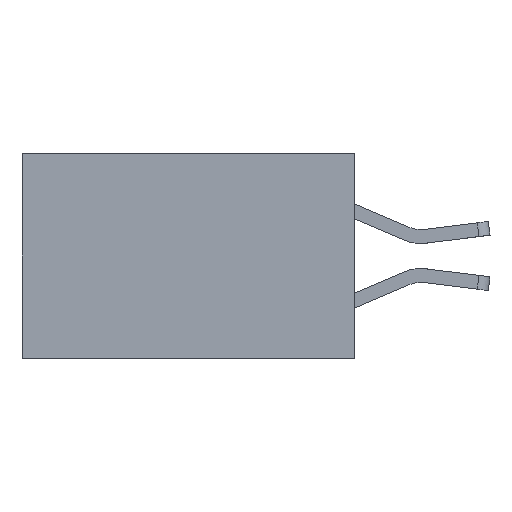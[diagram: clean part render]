
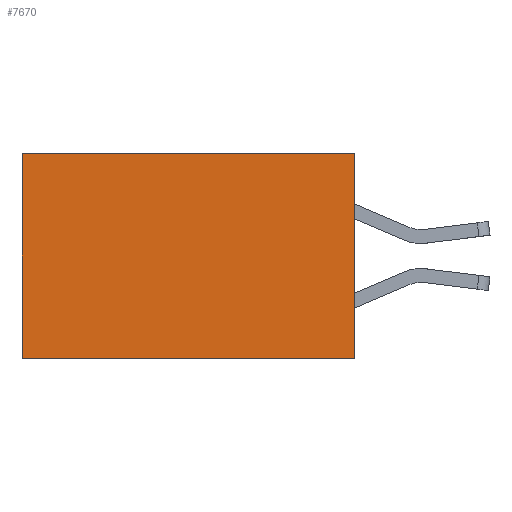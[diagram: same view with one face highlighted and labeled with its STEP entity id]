
A CAD part, left-side view. The second image highlights one B-rep face of the part: STEP entity #7670.
In plain terms, the highlighted planar face has unit normal (-1, 0, 0).
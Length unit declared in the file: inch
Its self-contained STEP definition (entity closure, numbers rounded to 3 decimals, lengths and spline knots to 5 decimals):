
#249 = ORIENTED_EDGE ( 'NONE', *, *, #6548, .T. ) ;
#794 = CARTESIAN_POINT ( 'NONE',  ( 0.298, 0., -0.37 ) ) ;
#805 = ORIENTED_EDGE ( 'NONE', *, *, #2614, .F. ) ;
#952 = VERTEX_POINT ( 'NONE', #5500 ) ;
#1514 = ORIENTED_EDGE ( 'NONE', *, *, #7347, .T. ) ;
#1633 = CARTESIAN_POINT ( 'NONE',  ( 0.298, 0.6, 0. ) ) ;
#2025 = CARTESIAN_POINT ( 'NONE',  ( 0.298, 0.6, 0. ) ) ;
#2119 = VECTOR ( 'NONE', #5147, 39.37008 ) ;
#2341 = VERTEX_POINT ( 'NONE', #1633 ) ;
#2614 = EDGE_CURVE ( 'NONE', #3844, #9428, #5479, .T. ) ;
#2723 = AXIS2_PLACEMENT_3D ( 'NONE', #10207, #2782, #7295 ) ;
#2782 = DIRECTION ( 'NONE',  ( 1., 0., 0. ) ) ;
#3348 = CARTESIAN_POINT ( 'NONE',  ( 0.298, 0., 0. ) ) ;
#3413 = CARTESIAN_POINT ( 'NONE',  ( 0.298, 0., -0.37 ) ) ;
#3664 = LINE ( 'NONE', #2025, #8101 ) ;
#3844 = VERTEX_POINT ( 'NONE', #4093 ) ;
#4093 = CARTESIAN_POINT ( 'NONE',  ( 0.298, 0., 0. ) ) ;
#5147 = DIRECTION ( 'NONE',  ( 0., 1., 0. ) ) ;
#5187 = DIRECTION ( 'NONE',  ( 0., 1., 0. ) ) ;
#5454 = DIRECTION ( 'NONE',  ( 0., 0., -1. ) ) ;
#5479 = LINE ( 'NONE', #3348, #9629 ) ;
#5481 = ORIENTED_EDGE ( 'NONE', *, *, #7722, .F. ) ;
#5500 = CARTESIAN_POINT ( 'NONE',  ( 0.298, 0.6, -0.37 ) ) ;
#6548 = EDGE_CURVE ( 'NONE', #3844, #2341, #8766, .T. ) ;
#6702 = VECTOR ( 'NONE', #5187, 39.37008 ) ;
#7295 = DIRECTION ( 'NONE',  ( 0., 0., -1. ) ) ;
#7347 = EDGE_CURVE ( 'NONE', #2341, #952, #3664, .T. ) ;
#7452 = FACE_OUTER_BOUND ( 'NONE', #9924, .T. ) ;
#7567 = DIRECTION ( 'NONE',  ( 0., 0., -1. ) ) ;
#7670 = ADVANCED_FACE ( 'NONE', ( #7452 ), #9814, .F. ) ;
#7722 = EDGE_CURVE ( 'NONE', #9428, #952, #8870, .T. ) ;
#8101 = VECTOR ( 'NONE', #5454, 39.37008 ) ;
#8766 = LINE ( 'NONE', #10384, #2119 ) ;
#8870 = LINE ( 'NONE', #794, #6702 ) ;
#9428 = VERTEX_POINT ( 'NONE', #3413 ) ;
#9629 = VECTOR ( 'NONE', #7567, 39.37008 ) ;
#9814 = PLANE ( 'NONE',  #2723 ) ;
#9924 = EDGE_LOOP ( 'NONE', ( #1514, #5481, #805, #249 ) ) ;
#10207 = CARTESIAN_POINT ( 'NONE',  ( 0.298, 0., 0. ) ) ;
#10384 = CARTESIAN_POINT ( 'NONE',  ( 0.298, 0., 0. ) ) ;
